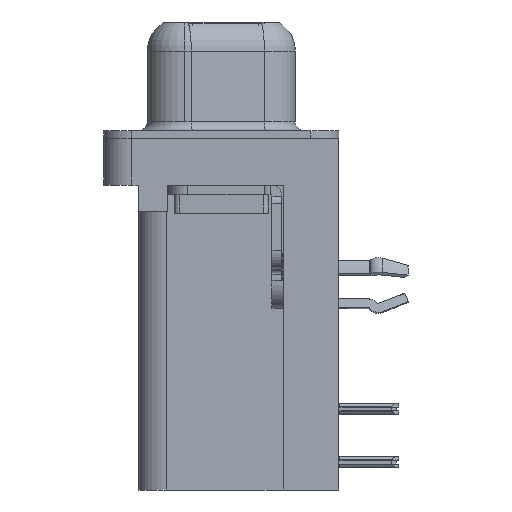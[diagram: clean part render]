
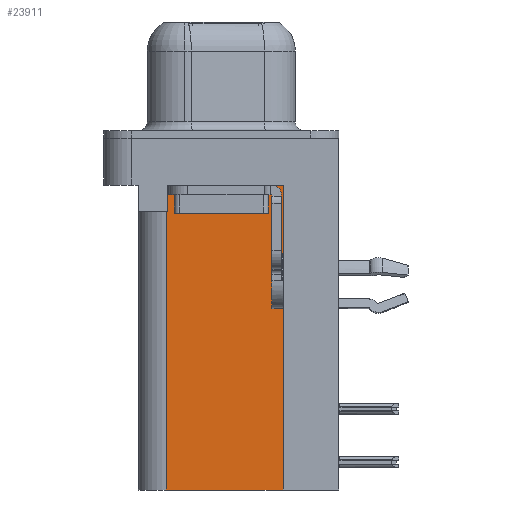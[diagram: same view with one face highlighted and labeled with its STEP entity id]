
A CAD part, left-side view. The second image highlights one B-rep face of the part: STEP entity #23911.
In plain terms, the highlighted planar face has unit normal (-1, 0, 0).
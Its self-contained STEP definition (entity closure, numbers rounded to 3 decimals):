
#1007 = DIRECTION ( 'NONE',  ( 0., 0., 1. ) ) ;
#1319 = CARTESIAN_POINT ( 'NONE',  ( 3.7, 2.895, -3.9 ) ) ;
#1841 = ORIENTED_EDGE ( 'NONE', *, *, #13728, .F. ) ;
#1885 = LINE ( 'NONE', #18831, #23671 ) ;
#2863 = VERTEX_POINT ( 'NONE', #20577 ) ;
#3105 = LINE ( 'NONE', #14546, #9877 ) ;
#4784 = AXIS2_PLACEMENT_3D ( 'NONE', #5132, #22857, #7692 ) ;
#5132 = CARTESIAN_POINT ( 'NONE',  ( 3.7, -3.295, -18.76 ) ) ;
#6631 = VECTOR ( 'NONE', #17424, 1000. ) ;
#6646 = CARTESIAN_POINT ( 'NONE',  ( 3.7, -3.295, -18.76 ) ) ;
#7150 = VERTEX_POINT ( 'NONE', #10128 ) ;
#7267 = CARTESIAN_POINT ( 'NONE',  ( 3.7, -3.295, -2.5 ) ) ;
#7692 = DIRECTION ( 'NONE',  ( 0., 1., 0. ) ) ;
#8967 = VERTEX_POINT ( 'NONE', #24789 ) ;
#9877 = VECTOR ( 'NONE', #29785, 1000. ) ;
#10128 = CARTESIAN_POINT ( 'NONE',  ( 3.7, 2.895, -3.9 ) ) ;
#10238 = LINE ( 'NONE', #16140, #22901 ) ;
#13232 = ORIENTED_EDGE ( 'NONE', *, *, #27068, .F. ) ;
#13345 = EDGE_CURVE ( 'NONE', #2863, #31362, #28883, .T. ) ;
#13728 = EDGE_CURVE ( 'NONE', #2863, #8967, #20108, .T. ) ;
#14546 = CARTESIAN_POINT ( 'NONE',  ( 3.7, 0., -3.9 ) ) ;
#14809 = VECTOR ( 'NONE', #21612, 1000. ) ;
#14867 = CARTESIAN_POINT ( 'NONE',  ( 3.7, -3.295, -18.76 ) ) ;
#15150 = PLANE ( 'NONE',  #4784 ) ;
#15317 = VECTOR ( 'NONE', #26907, 1000. ) ;
#15584 = LINE ( 'NONE', #1319, #14809 ) ;
#16140 = CARTESIAN_POINT ( 'NONE',  ( 3.7, 2.925, -18.76 ) ) ;
#16184 = EDGE_CURVE ( 'NONE', #17301, #7150, #15584, .T. ) ;
#17301 = VERTEX_POINT ( 'NONE', #28523 ) ;
#17424 = DIRECTION ( 'NONE',  ( 0., 1., 0. ) ) ;
#17551 = ORIENTED_EDGE ( 'NONE', *, *, #13345, .T. ) ;
#18831 = CARTESIAN_POINT ( 'NONE',  ( 3.7, -3.295, -2.5 ) ) ;
#20108 = LINE ( 'NONE', #14867, #6631 ) ;
#20577 = CARTESIAN_POINT ( 'NONE',  ( 3.7, -3.295, -18.76 ) ) ;
#21612 = DIRECTION ( 'NONE',  ( 0., 0., -1. ) ) ;
#22136 = ORIENTED_EDGE ( 'NONE', *, *, #16184, .T. ) ;
#22442 = ORIENTED_EDGE ( 'NONE', *, *, #27107, .T. ) ;
#22857 = DIRECTION ( 'NONE',  ( 1., 0., 0. ) ) ;
#22901 = VECTOR ( 'NONE', #1007, 1000. ) ;
#23671 = VECTOR ( 'NONE', #23907, 1000. ) ;
#23907 = DIRECTION ( 'NONE',  ( 0., 1., 0. ) ) ;
#23911 = ADVANCED_FACE ( 'NONE', ( #31009 ), #15150, .F. ) ;
#24789 = CARTESIAN_POINT ( 'NONE',  ( 3.7, 2.925, -18.76 ) ) ;
#26907 = DIRECTION ( 'NONE',  ( 0., 0., 1. ) ) ;
#27068 = EDGE_CURVE ( 'NONE', #8967, #29117, #10238, .T. ) ;
#27104 = ORIENTED_EDGE ( 'NONE', *, *, #32374, .T. ) ;
#27107 = EDGE_CURVE ( 'NONE', #31362, #17301, #1885, .T. ) ;
#28523 = CARTESIAN_POINT ( 'NONE',  ( 3.7, 2.895, -2.5 ) ) ;
#28883 = LINE ( 'NONE', #6646, #15317 ) ;
#29117 = VERTEX_POINT ( 'NONE', #31471 ) ;
#29785 = DIRECTION ( 'NONE',  ( 0., 1., 0. ) ) ;
#30526 = EDGE_LOOP ( 'NONE', ( #22442, #22136, #27104, #13232, #1841, #17551 ) ) ;
#31009 = FACE_OUTER_BOUND ( 'NONE', #30526, .T. ) ;
#31362 = VERTEX_POINT ( 'NONE', #7267 ) ;
#31471 = CARTESIAN_POINT ( 'NONE',  ( 3.7, 2.925, -3.9 ) ) ;
#32374 = EDGE_CURVE ( 'NONE', #7150, #29117, #3105, .T. ) ;
